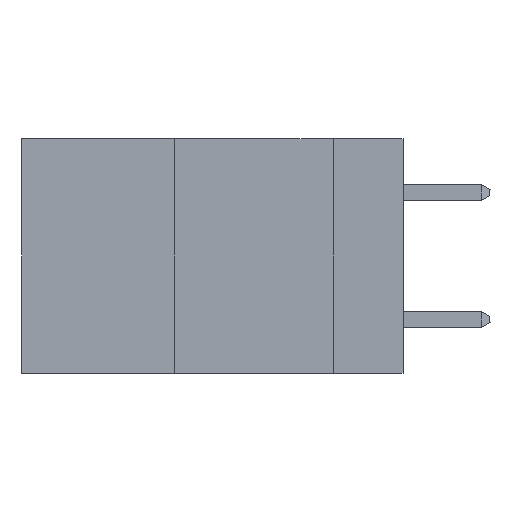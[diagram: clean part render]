
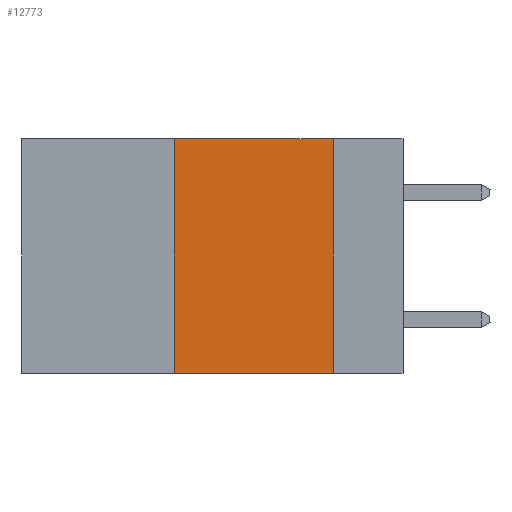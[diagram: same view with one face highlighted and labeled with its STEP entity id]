
A CAD part, left-side view. The second image highlights one B-rep face of the part: STEP entity #12773.
In plain terms, the highlighted planar face has unit normal (-1, 0, 0).
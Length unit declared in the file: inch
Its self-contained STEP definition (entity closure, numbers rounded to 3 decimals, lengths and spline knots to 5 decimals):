
#245 = AXIS2_PLACEMENT_3D ( 'NONE', #15218, #15124, #1875 ) ;
#392 = CARTESIAN_POINT ( 'NONE',  ( 0., 0.11, -0.37 ) ) ;
#407 = EDGE_CURVE ( 'NONE', #10660, #3420, #23849, .T. ) ;
#1875 = DIRECTION ( 'NONE',  ( 0., 0., -1. ) ) ;
#2385 = EDGE_CURVE ( 'NONE', #24092, #5370, #3680, .T. ) ;
#3420 = VERTEX_POINT ( 'NONE', #392 ) ;
#3680 = LINE ( 'NONE', #5105, #13778 ) ;
#4615 = EDGE_LOOP ( 'NONE', ( #24529, #7592, #19468, #21600 ) ) ;
#5105 = CARTESIAN_POINT ( 'NONE',  ( 0., 0.6, 0. ) ) ;
#5183 = VECTOR ( 'NONE', #12276, 39.37008 ) ;
#5309 = CARTESIAN_POINT ( 'NONE',  ( 0., 0.36, 0. ) ) ;
#5370 = VERTEX_POINT ( 'NONE', #17211 ) ;
#7410 = DIRECTION ( 'NONE',  ( 0., 0., 1. ) ) ;
#7592 = ORIENTED_EDGE ( 'NONE', *, *, #2385, .F. ) ;
#9770 = FACE_OUTER_BOUND ( 'NONE', #4615, .T. ) ;
#10361 = CARTESIAN_POINT ( 'NONE',  ( 0., 0.36, -0.37 ) ) ;
#10660 = VERTEX_POINT ( 'NONE', #10361 ) ;
#11508 = VECTOR ( 'NONE', #7410, 39.37008 ) ;
#11991 = DIRECTION ( 'NONE',  ( 0., -1., 0. ) ) ;
#12276 = DIRECTION ( 'NONE',  ( 0., -1., 0. ) ) ;
#12406 = CARTESIAN_POINT ( 'NONE',  ( 0., 0.11, 0. ) ) ;
#12604 = DIRECTION ( 'NONE',  ( 0., 0., -1. ) ) ;
#12773 = ADVANCED_FACE ( 'NONE', ( #9770 ), #21663, .F. ) ;
#13778 = VECTOR ( 'NONE', #11991, 39.37008 ) ;
#15124 = DIRECTION ( 'NONE',  ( 1., 0., 0. ) ) ;
#15218 = CARTESIAN_POINT ( 'NONE',  ( 0., 0.6, 0. ) ) ;
#17211 = CARTESIAN_POINT ( 'NONE',  ( 0., 0.11, 0. ) ) ;
#17599 = VECTOR ( 'NONE', #12604, 39.37008 ) ;
#17852 = CARTESIAN_POINT ( 'NONE',  ( 0., 0.36, 0. ) ) ;
#19468 = ORIENTED_EDGE ( 'NONE', *, *, #25864, .F. ) ;
#20941 = CARTESIAN_POINT ( 'NONE',  ( 0., 0.6, -0.37 ) ) ;
#21011 = LINE ( 'NONE', #12406, #17599 ) ;
#21079 = EDGE_CURVE ( 'NONE', #5370, #3420, #21011, .T. ) ;
#21600 = ORIENTED_EDGE ( 'NONE', *, *, #407, .T. ) ;
#21663 = PLANE ( 'NONE',  #245 ) ;
#23849 = LINE ( 'NONE', #20941, #5183 ) ;
#24092 = VERTEX_POINT ( 'NONE', #17852 ) ;
#24529 = ORIENTED_EDGE ( 'NONE', *, *, #21079, .F. ) ;
#25864 = EDGE_CURVE ( 'NONE', #10660, #24092, #27696, .T. ) ;
#27696 = LINE ( 'NONE', #5309, #11508 ) ;
